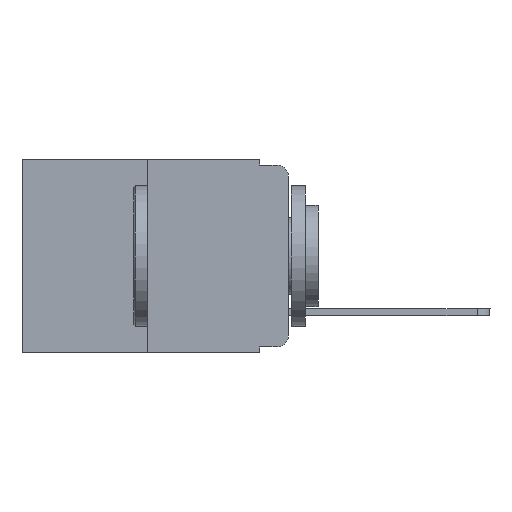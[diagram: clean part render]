
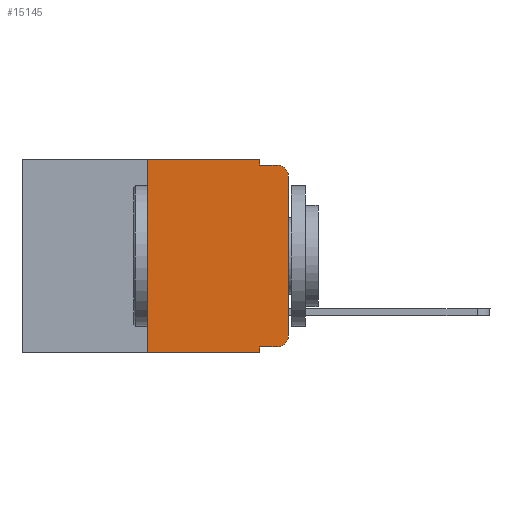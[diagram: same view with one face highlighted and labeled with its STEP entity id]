
A CAD part, left-side view. The second image highlights one B-rep face of the part: STEP entity #15145.
In plain terms, the highlighted planar face has unit normal (-1, 0, 0).
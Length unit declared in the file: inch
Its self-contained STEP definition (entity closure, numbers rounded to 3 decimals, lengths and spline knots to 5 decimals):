
#132 = EDGE_CURVE ( 'NONE', #25768, #9916, #11379, .T. ) ;
#371 = VERTEX_POINT ( 'NONE', #6773 ) ;
#1617 = CARTESIAN_POINT ( 'NONE',  ( 0., 0.02, -0.01 ) ) ;
#1624 = VECTOR ( 'NONE', #8230, 39.37008 ) ;
#1713 = ORIENTED_EDGE ( 'NONE', *, *, #25355, .T. ) ;
#2121 = LINE ( 'NONE', #12888, #9403 ) ;
#2184 = DIRECTION ( 'NONE',  ( -1., 0., 0. ) ) ;
#2518 = VERTEX_POINT ( 'NONE', #17613 ) ;
#3079 = CARTESIAN_POINT ( 'NONE',  ( 0., 0.25, 0. ) ) ;
#4381 = DIRECTION ( 'NONE',  ( 0., -1., 0. ) ) ;
#4437 = VECTOR ( 'NONE', #13767, 39.37008 ) ;
#4857 = VERTEX_POINT ( 'NONE', #15579 ) ;
#5048 = DIRECTION ( 'NONE',  ( 0., 0., -1. ) ) ;
#5796 = EDGE_CURVE ( 'NONE', #11917, #371, #6652, .T. ) ;
#6652 = LINE ( 'NONE', #23778, #4437 ) ;
#6773 = CARTESIAN_POINT ( 'NONE',  ( 0., 0.051, -0.343 ) ) ;
#6779 = CARTESIAN_POINT ( 'NONE',  ( 0., 0.25, 0. ) ) ;
#7536 = CARTESIAN_POINT ( 'NONE',  ( 0., 0.051, -0.01 ) ) ;
#7998 = ORIENTED_EDGE ( 'NONE', *, *, #5796, .F. ) ;
#8032 = LINE ( 'NONE', #7536, #22143 ) ;
#8072 = ORIENTED_EDGE ( 'NONE', *, *, #15766, .F. ) ;
#8078 = CARTESIAN_POINT ( 'NONE',  ( 0., 0.051, -0.01 ) ) ;
#8230 = DIRECTION ( 'NONE',  ( 0., -1., 0. ) ) ;
#8476 = LINE ( 'NONE', #22054, #10806 ) ;
#9403 = VECTOR ( 'NONE', #5048, 39.37008 ) ;
#9474 = LINE ( 'NONE', #25785, #20186 ) ;
#9606 = CARTESIAN_POINT ( 'NONE',  ( 0., 0., -0.03 ) ) ;
#9696 = VERTEX_POINT ( 'NONE', #22921 ) ;
#9916 = VERTEX_POINT ( 'NONE', #1617 ) ;
#9922 = DIRECTION ( 'NONE',  ( -1., 0., 0. ) ) ;
#10162 = ORIENTED_EDGE ( 'NONE', *, *, #25059, .T. ) ;
#10481 = CARTESIAN_POINT ( 'NONE',  ( 0., 0.02, -0.313 ) ) ;
#10484 = VERTEX_POINT ( 'NONE', #3079 ) ;
#10806 = VECTOR ( 'NONE', #26037, 39.37008 ) ;
#10817 = DIRECTION ( 'NONE',  ( 0., 0., 1. ) ) ;
#11167 = ORIENTED_EDGE ( 'NONE', *, *, #17750, .F. ) ;
#11379 = CIRCLE ( 'NONE', #11998, 0.02 ) ;
#11467 = VECTOR ( 'NONE', #4381, 39.37008 ) ;
#11917 = VERTEX_POINT ( 'NONE', #25488 ) ;
#11985 = DIRECTION ( 'NONE',  ( 0., 0., -1. ) ) ;
#11998 = AXIS2_PLACEMENT_3D ( 'NONE', #19853, #9922, #11985 ) ;
#12292 = EDGE_CURVE ( 'NONE', #24895, #10484, #14148, .T. ) ;
#12379 = CARTESIAN_POINT ( 'NONE',  ( 0., 0.051, -0.333 ) ) ;
#12469 = CARTESIAN_POINT ( 'NONE',  ( 0., 0.25, -0.343 ) ) ;
#12792 = CIRCLE ( 'NONE', #19321, 0.02 ) ;
#12816 = EDGE_CURVE ( 'NONE', #4857, #24352, #2121, .T. ) ;
#12888 = CARTESIAN_POINT ( 'NONE',  ( 0., 0.051, 0. ) ) ;
#13613 = ORIENTED_EDGE ( 'NONE', *, *, #12816, .F. ) ;
#13669 = DIRECTION ( 'NONE',  ( 0., -1., 0. ) ) ;
#13767 = DIRECTION ( 'NONE',  ( 0., 0., -1. ) ) ;
#13887 = LINE ( 'NONE', #18259, #1624 ) ;
#14148 = LINE ( 'NONE', #6779, #20177 ) ;
#14330 = DIRECTION ( 'NONE',  ( 0., 0., -1. ) ) ;
#15145 = ADVANCED_FACE ( 'NONE', ( #21255 ), #20352, .F. ) ;
#15579 = CARTESIAN_POINT ( 'NONE',  ( 0., 0.051, 0. ) ) ;
#15766 = EDGE_CURVE ( 'NONE', #24352, #9916, #8032, .T. ) ;
#16261 = DIRECTION ( 'NONE',  ( 0., 0., -1. ) ) ;
#16484 = EDGE_CURVE ( 'NONE', #11917, #2518, #16796, .T. ) ;
#16796 = LINE ( 'NONE', #12379, #11467 ) ;
#17613 = CARTESIAN_POINT ( 'NONE',  ( 0., 0.02, -0.333 ) ) ;
#17722 = ORIENTED_EDGE ( 'NONE', *, *, #132, .T. ) ;
#17750 = EDGE_CURVE ( 'NONE', #10484, #4857, #13887, .T. ) ;
#18223 = EDGE_CURVE ( 'NONE', #24895, #371, #9474, .T. ) ;
#18259 = CARTESIAN_POINT ( 'NONE',  ( 0., 0.473, 0. ) ) ;
#18488 = DIRECTION ( 'NONE',  ( 1., 0., 0. ) ) ;
#19221 = EDGE_LOOP ( 'NONE', ( #10162, #17722, #8072, #13613, #11167, #21799, #22548, #7998, #19990, #1713 ) ) ;
#19321 = AXIS2_PLACEMENT_3D ( 'NONE', #10481, #2184, #16261 ) ;
#19724 = DIRECTION ( 'NONE',  ( 0., -1., 0. ) ) ;
#19853 = CARTESIAN_POINT ( 'NONE',  ( 0., 0.02, -0.03 ) ) ;
#19990 = ORIENTED_EDGE ( 'NONE', *, *, #16484, .T. ) ;
#20177 = VECTOR ( 'NONE', #10817, 39.37008 ) ;
#20186 = VECTOR ( 'NONE', #19724, 39.37008 ) ;
#20352 = PLANE ( 'NONE',  #20847 ) ;
#20847 = AXIS2_PLACEMENT_3D ( 'NONE', #22485, #18488, #14330 ) ;
#21255 = FACE_OUTER_BOUND ( 'NONE', #19221, .T. ) ;
#21799 = ORIENTED_EDGE ( 'NONE', *, *, #12292, .F. ) ;
#22054 = CARTESIAN_POINT ( 'NONE',  ( 0., 0., 0. ) ) ;
#22143 = VECTOR ( 'NONE', #13669, 39.37008 ) ;
#22485 = CARTESIAN_POINT ( 'NONE',  ( 0., 0.473, 0. ) ) ;
#22548 = ORIENTED_EDGE ( 'NONE', *, *, #18223, .T. ) ;
#22921 = CARTESIAN_POINT ( 'NONE',  ( 0., 0., -0.313 ) ) ;
#23778 = CARTESIAN_POINT ( 'NONE',  ( 0., 0.051, 0. ) ) ;
#24352 = VERTEX_POINT ( 'NONE', #8078 ) ;
#24895 = VERTEX_POINT ( 'NONE', #12469 ) ;
#25059 = EDGE_CURVE ( 'NONE', #9696, #25768, #8476, .T. ) ;
#25355 = EDGE_CURVE ( 'NONE', #2518, #9696, #12792, .T. ) ;
#25488 = CARTESIAN_POINT ( 'NONE',  ( 0., 0.051, -0.333 ) ) ;
#25768 = VERTEX_POINT ( 'NONE', #9606 ) ;
#25785 = CARTESIAN_POINT ( 'NONE',  ( 0., 0.473, -0.343 ) ) ;
#26037 = DIRECTION ( 'NONE',  ( 0., 0., 1. ) ) ;
